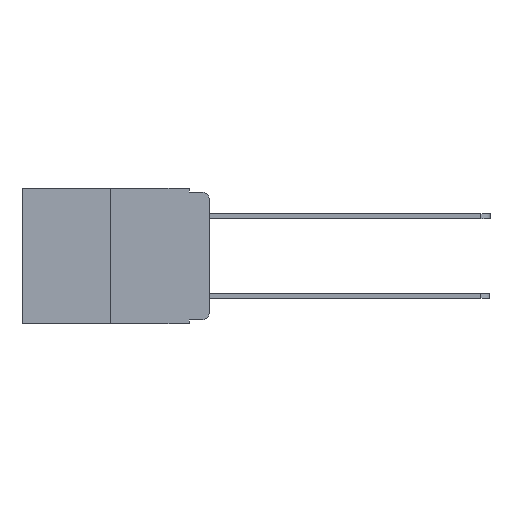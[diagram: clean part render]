
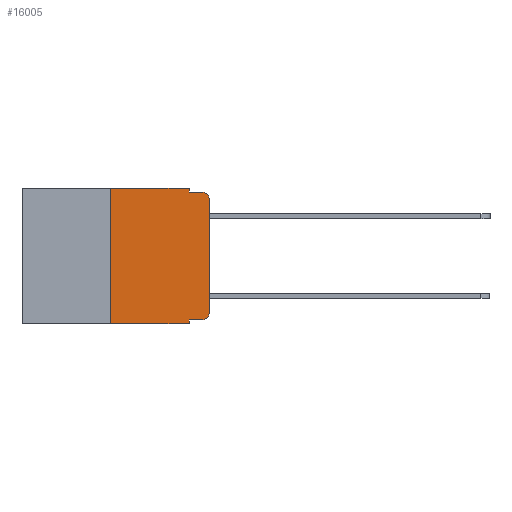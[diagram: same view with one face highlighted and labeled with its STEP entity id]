
A CAD part, left-side view. The second image highlights one B-rep face of the part: STEP entity #16005.
In plain terms, the highlighted planar face has unit normal (-1, 0, 0).
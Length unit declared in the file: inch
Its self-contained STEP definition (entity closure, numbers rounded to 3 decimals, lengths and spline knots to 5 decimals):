
#167 = ORIENTED_EDGE ( 'NONE', *, *, #17655, .T. ) ;
#1193 = DIRECTION ( 'NONE',  ( 0., 0., 1. ) ) ;
#1258 = VERTEX_POINT ( 'NONE', #11641 ) ;
#1456 = VERTEX_POINT ( 'NONE', #2759 ) ;
#1460 = VERTEX_POINT ( 'NONE', #6022 ) ;
#1628 = DIRECTION ( 'NONE',  ( 0., -1., 0. ) ) ;
#2010 = VERTEX_POINT ( 'NONE', #9365 ) ;
#2411 = CARTESIAN_POINT ( 'NONE',  ( 0., 0.051, -0.01 ) ) ;
#2714 = LINE ( 'NONE', #2411, #14919 ) ;
#2759 = CARTESIAN_POINT ( 'NONE',  ( 0., 0.25, -0.343 ) ) ;
#2927 = EDGE_CURVE ( 'NONE', #1456, #9244, #20309, .T. ) ;
#3152 = ORIENTED_EDGE ( 'NONE', *, *, #18721, .T. ) ;
#3382 = ORIENTED_EDGE ( 'NONE', *, *, #2927, .F. ) ;
#3501 = EDGE_CURVE ( 'NONE', #9244, #10034, #17868, .T. ) ;
#3631 = DIRECTION ( 'NONE',  ( 0., 0., -1. ) ) ;
#3903 = CARTESIAN_POINT ( 'NONE',  ( 0., 0.02, -0.01 ) ) ;
#4014 = EDGE_CURVE ( 'NONE', #10034, #2010, #15694, .T. ) ;
#4181 = CARTESIAN_POINT ( 'NONE',  ( 0., 0.02, -0.333 ) ) ;
#4263 = CARTESIAN_POINT ( 'NONE',  ( 0., 0.051, 0. ) ) ;
#4313 = ORIENTED_EDGE ( 'NONE', *, *, #9702, .T. ) ;
#4963 = AXIS2_PLACEMENT_3D ( 'NONE', #16504, #6641, #18102 ) ;
#5136 = EDGE_CURVE ( 'NONE', #2010, #17679, #2714, .T. ) ;
#5222 = CARTESIAN_POINT ( 'NONE',  ( 0., 0.473, 0. ) ) ;
#5682 = VERTEX_POINT ( 'NONE', #10813 ) ;
#5760 = DIRECTION ( 'NONE',  ( 0., -1., 0. ) ) ;
#6022 = CARTESIAN_POINT ( 'NONE',  ( 0., 0.051, -0.333 ) ) ;
#6309 = VECTOR ( 'NONE', #5760, 39.37008 ) ;
#6476 = CIRCLE ( 'NONE', #4963, 0.02 ) ;
#6481 = ORIENTED_EDGE ( 'NONE', *, *, #8522, .T. ) ;
#6641 = DIRECTION ( 'NONE',  ( -1., 0., 0. ) ) ;
#7235 = DIRECTION ( 'NONE',  ( -1., 0., 0. ) ) ;
#7540 = DIRECTION ( 'NONE',  ( 0., 0., -1. ) ) ;
#7663 = EDGE_LOOP ( 'NONE', ( #4313, #6481, #8239, #8289, #16499, #3382, #18524, #9472, #3152, #167 ) ) ;
#7911 = VECTOR ( 'NONE', #12121, 39.37008 ) ;
#8239 = ORIENTED_EDGE ( 'NONE', *, *, #5136, .F. ) ;
#8270 = CARTESIAN_POINT ( 'NONE',  ( 0., 0.473, 0. ) ) ;
#8289 = ORIENTED_EDGE ( 'NONE', *, *, #4014, .F. ) ;
#8522 = EDGE_CURVE ( 'NONE', #5682, #17679, #6476, .T. ) ;
#8571 = VECTOR ( 'NONE', #1628, 39.37008 ) ;
#8832 = CARTESIAN_POINT ( 'NONE',  ( 0., 0.051, -0.343 ) ) ;
#9199 = VECTOR ( 'NONE', #21220, 39.37008 ) ;
#9244 = VERTEX_POINT ( 'NONE', #14971 ) ;
#9365 = CARTESIAN_POINT ( 'NONE',  ( 0., 0.051, -0.01 ) ) ;
#9472 = ORIENTED_EDGE ( 'NONE', *, *, #19746, .F. ) ;
#9528 = CIRCLE ( 'NONE', #20714, 0.02 ) ;
#9702 = EDGE_CURVE ( 'NONE', #1258, #5682, #11195, .T. ) ;
#10034 = VERTEX_POINT ( 'NONE', #13655 ) ;
#10813 = CARTESIAN_POINT ( 'NONE',  ( 0., 0., -0.03 ) ) ;
#11195 = LINE ( 'NONE', #12936, #15499 ) ;
#11420 = VECTOR ( 'NONE', #12039, 39.37008 ) ;
#11641 = CARTESIAN_POINT ( 'NONE',  ( 0., 0., -0.313 ) ) ;
#11956 = CARTESIAN_POINT ( 'NONE',  ( 0., 0.25, 0. ) ) ;
#11982 = PLANE ( 'NONE',  #19933 ) ;
#11985 = CARTESIAN_POINT ( 'NONE',  ( 0., 0.051, 0. ) ) ;
#12039 = DIRECTION ( 'NONE',  ( 0., 0., -1. ) ) ;
#12121 = DIRECTION ( 'NONE',  ( 0., 0., 1. ) ) ;
#12936 = CARTESIAN_POINT ( 'NONE',  ( 0., 0., 0. ) ) ;
#13109 = VERTEX_POINT ( 'NONE', #8832 ) ;
#13365 = CARTESIAN_POINT ( 'NONE',  ( 0., 0.473, -0.343 ) ) ;
#13396 = CARTESIAN_POINT ( 'NONE',  ( 0., 0.051, -0.333 ) ) ;
#13606 = LINE ( 'NONE', #13396, #9199 ) ;
#13655 = CARTESIAN_POINT ( 'NONE',  ( 0., 0.051, 0. ) ) ;
#13657 = DIRECTION ( 'NONE',  ( 1., 0., 0. ) ) ;
#14293 = LINE ( 'NONE', #4263, #17987 ) ;
#14919 = VECTOR ( 'NONE', #15629, 39.37008 ) ;
#14971 = CARTESIAN_POINT ( 'NONE',  ( 0., 0.25, 0. ) ) ;
#15499 = VECTOR ( 'NONE', #1193, 39.37008 ) ;
#15629 = DIRECTION ( 'NONE',  ( 0., -1., 0. ) ) ;
#15694 = LINE ( 'NONE', #11985, #11420 ) ;
#16005 = ADVANCED_FACE ( 'NONE', ( #16852 ), #11982, .F. ) ;
#16204 = VERTEX_POINT ( 'NONE', #4181 ) ;
#16499 = ORIENTED_EDGE ( 'NONE', *, *, #3501, .F. ) ;
#16504 = CARTESIAN_POINT ( 'NONE',  ( 0., 0.02, -0.03 ) ) ;
#16852 = FACE_OUTER_BOUND ( 'NONE', #7663, .T. ) ;
#17062 = CARTESIAN_POINT ( 'NONE',  ( 0., 0.02, -0.313 ) ) ;
#17655 = EDGE_CURVE ( 'NONE', #16204, #1258, #9528, .T. ) ;
#17679 = VERTEX_POINT ( 'NONE', #3903 ) ;
#17868 = LINE ( 'NONE', #8270, #6309 ) ;
#17987 = VECTOR ( 'NONE', #7540, 39.37008 ) ;
#18102 = DIRECTION ( 'NONE',  ( 0., 0., -1. ) ) ;
#18524 = ORIENTED_EDGE ( 'NONE', *, *, #20017, .T. ) ;
#18673 = DIRECTION ( 'NONE',  ( 0., 0., -1. ) ) ;
#18721 = EDGE_CURVE ( 'NONE', #1460, #16204, #13606, .T. ) ;
#19746 = EDGE_CURVE ( 'NONE', #1460, #13109, #14293, .T. ) ;
#19933 = AXIS2_PLACEMENT_3D ( 'NONE', #5222, #13657, #3631 ) ;
#20017 = EDGE_CURVE ( 'NONE', #1456, #13109, #20859, .T. ) ;
#20309 = LINE ( 'NONE', #11956, #7911 ) ;
#20714 = AXIS2_PLACEMENT_3D ( 'NONE', #17062, #7235, #18673 ) ;
#20859 = LINE ( 'NONE', #13365, #8571 ) ;
#21220 = DIRECTION ( 'NONE',  ( 0., -1., 0. ) ) ;
